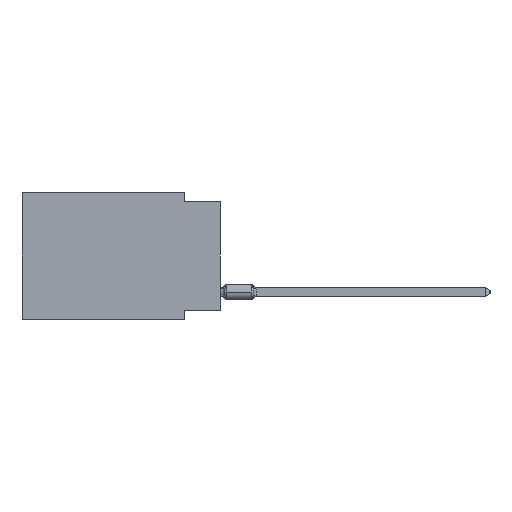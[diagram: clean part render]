
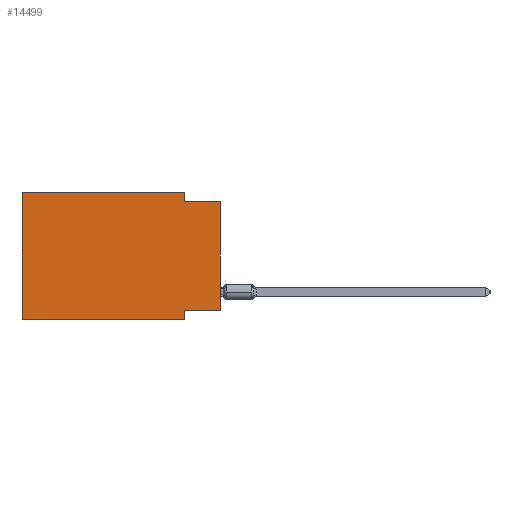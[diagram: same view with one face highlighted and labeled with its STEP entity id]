
A CAD part, left-side view. The second image highlights one B-rep face of the part: STEP entity #14499.
In plain terms, the highlighted planar face has unit normal (-1, 0, 0).
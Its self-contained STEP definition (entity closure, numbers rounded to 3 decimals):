
#55 = VERTEX_POINT ( 'NONE', #9060 ) ;
#681 = VERTEX_POINT ( 'NONE', #4875 ) ;
#1666 = DIRECTION ( 'NONE',  ( 0., 0., -1. ) ) ;
#2112 = DIRECTION ( 'NONE',  ( 0., 0., -1. ) ) ;
#2741 = VECTOR ( 'NONE', #2112, 1000. ) ;
#2824 = CARTESIAN_POINT ( 'NONE',  ( 0., 2.54, -8.89 ) ) ;
#2977 = CARTESIAN_POINT ( 'NONE',  ( 0., 0., -8.255 ) ) ;
#3880 = VECTOR ( 'NONE', #45778, 1000. ) ;
#3904 = AXIS2_PLACEMENT_3D ( 'NONE', #10816, #20525, #1666 ) ;
#4875 = CARTESIAN_POINT ( 'NONE',  ( 0., 0., -0.635 ) ) ;
#5488 = VECTOR ( 'NONE', #20667, 1000. ) ;
#5659 = EDGE_CURVE ( 'NONE', #55, #52894, #21149, .T. ) ;
#6379 = PLANE ( 'NONE',  #3904 ) ;
#6957 = LINE ( 'NONE', #2824, #56304 ) ;
#7517 = EDGE_CURVE ( 'NONE', #20066, #55, #27811, .T. ) ;
#7577 = CARTESIAN_POINT ( 'NONE',  ( 0., 13.97, 0. ) ) ;
#9049 = LINE ( 'NONE', #22618, #29479 ) ;
#9060 = CARTESIAN_POINT ( 'NONE',  ( 0., 13.97, 0. ) ) ;
#10005 = VECTOR ( 'NONE', #41063, 1000. ) ;
#10816 = CARTESIAN_POINT ( 'NONE',  ( 0., 13.97, 0. ) ) ;
#11630 = ORIENTED_EDGE ( 'NONE', *, *, #38981, .F. ) ;
#11921 = EDGE_CURVE ( 'NONE', #30042, #46921, #19858, .T. ) ;
#12115 = CARTESIAN_POINT ( 'NONE',  ( 0., 0., 0. ) ) ;
#12957 = EDGE_CURVE ( 'NONE', #46921, #52177, #6957, .T. ) ;
#13083 = CARTESIAN_POINT ( 'NONE',  ( 0., 13.97, -8.89 ) ) ;
#13123 = CARTESIAN_POINT ( 'NONE',  ( 0., 13.97, -8.89 ) ) ;
#13546 = VECTOR ( 'NONE', #29577, 1000. ) ;
#14268 = CARTESIAN_POINT ( 'NONE',  ( 0., 13.97, 0. ) ) ;
#14499 = ADVANCED_FACE ( 'NONE', ( #51474 ), #6379, .F. ) ;
#16999 = EDGE_CURVE ( 'NONE', #20066, #52177, #36347, .T. ) ;
#17356 = CARTESIAN_POINT ( 'NONE',  ( 0., 2.54, -0.635 ) ) ;
#18487 = DIRECTION ( 'NONE',  ( 0., -1., 0. ) ) ;
#19858 = LINE ( 'NONE', #33410, #13546 ) ;
#20066 = VERTEX_POINT ( 'NONE', #13123 ) ;
#20525 = DIRECTION ( 'NONE',  ( 1., 0., 0. ) ) ;
#20667 = DIRECTION ( 'NONE',  ( 0., 0., 1. ) ) ;
#21149 = LINE ( 'NONE', #7577, #56374 ) ;
#21724 = DIRECTION ( 'NONE',  ( 0., -1., 0. ) ) ;
#22618 = CARTESIAN_POINT ( 'NONE',  ( 0., 0., -0.635 ) ) ;
#23099 = ORIENTED_EDGE ( 'NONE', *, *, #16999, .T. ) ;
#27094 = ORIENTED_EDGE ( 'NONE', *, *, #30948, .F. ) ;
#27811 = LINE ( 'NONE', #14268, #3880 ) ;
#29479 = VECTOR ( 'NONE', #18487, 1000. ) ;
#29577 = DIRECTION ( 'NONE',  ( 0., 1., 0. ) ) ;
#29814 = LINE ( 'NONE', #47212, #2741 ) ;
#30042 = VERTEX_POINT ( 'NONE', #2977 ) ;
#30948 = EDGE_CURVE ( 'NONE', #42892, #681, #9049, .T. ) ;
#33410 = CARTESIAN_POINT ( 'NONE',  ( 0., 0., -8.255 ) ) ;
#33530 = ORIENTED_EDGE ( 'NONE', *, *, #36857, .T. ) ;
#33876 = ORIENTED_EDGE ( 'NONE', *, *, #7517, .F. ) ;
#34953 = DIRECTION ( 'NONE',  ( 0., 0., -1. ) ) ;
#35092 = CARTESIAN_POINT ( 'NONE',  ( 0., 2.54, 0. ) ) ;
#36347 = LINE ( 'NONE', #13083, #10005 ) ;
#36857 = EDGE_CURVE ( 'NONE', #30042, #681, #38946, .T. ) ;
#38946 = LINE ( 'NONE', #12115, #5488 ) ;
#38981 = EDGE_CURVE ( 'NONE', #52894, #42892, #29814, .T. ) ;
#40261 = EDGE_LOOP ( 'NONE', ( #33530, #27094, #11630, #54085, #33876, #23099, #48831, #54655 ) ) ;
#41063 = DIRECTION ( 'NONE',  ( 0., -1., 0. ) ) ;
#42892 = VERTEX_POINT ( 'NONE', #17356 ) ;
#44320 = CARTESIAN_POINT ( 'NONE',  ( 0., 2.54, -8.255 ) ) ;
#45778 = DIRECTION ( 'NONE',  ( 0., 0., 1. ) ) ;
#46921 = VERTEX_POINT ( 'NONE', #44320 ) ;
#47212 = CARTESIAN_POINT ( 'NONE',  ( 0., 2.54, 0. ) ) ;
#48831 = ORIENTED_EDGE ( 'NONE', *, *, #12957, .F. ) ;
#51474 = FACE_OUTER_BOUND ( 'NONE', #40261, .T. ) ;
#52177 = VERTEX_POINT ( 'NONE', #52274 ) ;
#52274 = CARTESIAN_POINT ( 'NONE',  ( 0., 2.54, -8.89 ) ) ;
#52894 = VERTEX_POINT ( 'NONE', #35092 ) ;
#54085 = ORIENTED_EDGE ( 'NONE', *, *, #5659, .F. ) ;
#54655 = ORIENTED_EDGE ( 'NONE', *, *, #11921, .F. ) ;
#56304 = VECTOR ( 'NONE', #34953, 1000. ) ;
#56374 = VECTOR ( 'NONE', #21724, 1000. ) ;
